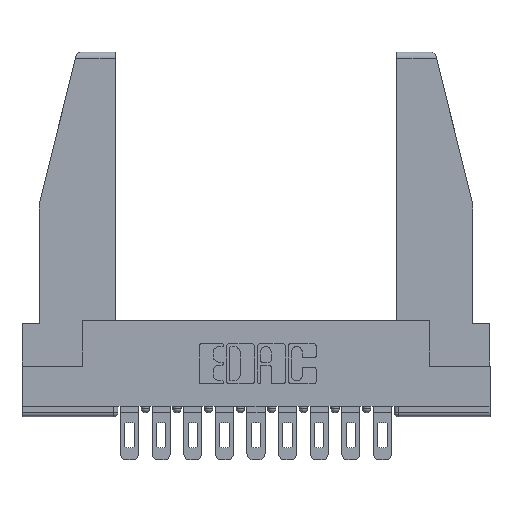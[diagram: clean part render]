
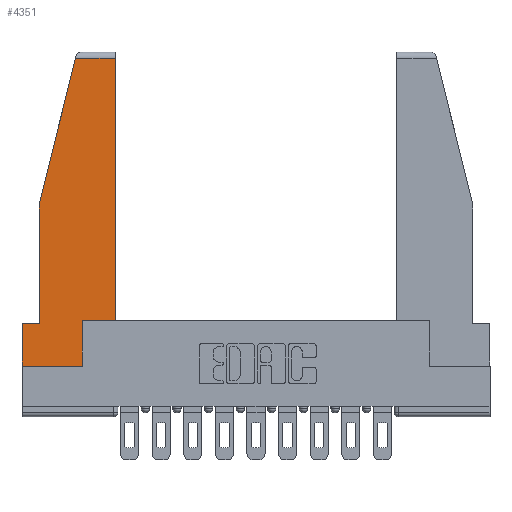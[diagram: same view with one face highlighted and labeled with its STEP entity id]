
A CAD part, top view. The second image highlights one B-rep face of the part: STEP entity #4351.
In plain terms, the highlighted planar face has unit normal (0, 0, 1).
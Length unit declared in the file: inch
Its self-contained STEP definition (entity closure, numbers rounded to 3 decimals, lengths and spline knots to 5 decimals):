
#62 = LINE ( 'NONE', #11621, #13755 ) ;
#148 = CARTESIAN_POINT ( 'NONE',  ( 0.2636, 1.52, 0. ) ) ;
#580 = CARTESIAN_POINT ( 'NONE',  ( 0., 1.52, 0. ) ) ;
#766 = LINE ( 'NONE', #9977, #7907 ) ;
#957 = LINE ( 'NONE', #4331, #13274 ) ;
#1027 = ORIENTED_EDGE ( 'NONE', *, *, #6216, .T. ) ;
#1059 = VERTEX_POINT ( 'NONE', #148 ) ;
#1178 = DIRECTION ( 'NONE',  ( 0., 1., 0. ) ) ;
#1854 = VERTEX_POINT ( 'NONE', #5735 ) ;
#1939 = CARTESIAN_POINT ( 'NONE',  ( 0., 0.21, 0. ) ) ;
#2094 = LINE ( 'NONE', #1939, #12218 ) ;
#2110 = EDGE_LOOP ( 'NONE', ( #8603, #5921, #12155, #1027, #12342, #12570, #11087, #5891, #13607 ) ) ;
#2282 = DIRECTION ( 'NONE',  ( 0., 1., 0. ) ) ;
#3157 = DIRECTION ( 'NONE',  ( -1., 0., 0. ) ) ;
#3195 = DIRECTION ( 'NONE',  ( 0., -1., 0. ) ) ;
#3197 = VECTOR ( 'NONE', #13126, 39.37008 ) ;
#3255 = PLANE ( 'NONE',  #10807 ) ;
#3324 = DIRECTION ( 'NONE',  ( -0.239, -0.971, 0. ) ) ;
#3366 = VERTEX_POINT ( 'NONE', #14363 ) ;
#3514 = CARTESIAN_POINT ( 'NONE',  ( 0.461, 0.223, 0. ) ) ;
#3780 = VERTEX_POINT ( 'NONE', #7477 ) ;
#3920 = VERTEX_POINT ( 'NONE', #4432 ) ;
#3982 = EDGE_CURVE ( 'NONE', #3780, #3366, #766, .T. ) ;
#4331 = CARTESIAN_POINT ( 'NONE',  ( 0.271, 1.55, 0. ) ) ;
#4351 = ADVANCED_FACE ( 'NONE', ( #12247 ), #3255, .T. ) ;
#4432 = CARTESIAN_POINT ( 'NONE',  ( 0.086, 0.8, 0. ) ) ;
#4512 = EDGE_CURVE ( 'NONE', #1854, #13811, #62, .T. ) ;
#4668 = VERTEX_POINT ( 'NONE', #13221 ) ;
#5735 = CARTESIAN_POINT ( 'NONE',  ( 0.297, 0.223, 0. ) ) ;
#5763 = VERTEX_POINT ( 'NONE', #11173 ) ;
#5773 = CARTESIAN_POINT ( 'NONE',  ( 0.461, 0.223, 0. ) ) ;
#5867 = VECTOR ( 'NONE', #13600, 39.37008 ) ;
#5891 = ORIENTED_EDGE ( 'NONE', *, *, #8280, .T. ) ;
#5921 = ORIENTED_EDGE ( 'NONE', *, *, #11559, .T. ) ;
#5927 = DIRECTION ( 'NONE',  ( 1., 0., 0. ) ) ;
#5994 = LINE ( 'NONE', #12912, #12396 ) ;
#6216 = EDGE_CURVE ( 'NONE', #3920, #4668, #9172, .T. ) ;
#6544 = DIRECTION ( 'NONE',  ( 1., 0., 0. ) ) ;
#6897 = EDGE_CURVE ( 'NONE', #1059, #3920, #957, .T. ) ;
#7081 = VECTOR ( 'NONE', #2282, 39.37008 ) ;
#7477 = CARTESIAN_POINT ( 'NONE',  ( 0., 0.21, 0. ) ) ;
#7907 = VECTOR ( 'NONE', #3195, 39.37008 ) ;
#8280 = EDGE_CURVE ( 'NONE', #14817, #1854, #5994, .T. ) ;
#8603 = ORIENTED_EDGE ( 'NONE', *, *, #9186, .T. ) ;
#9172 = LINE ( 'NONE', #13759, #10819 ) ;
#9186 = EDGE_CURVE ( 'NONE', #13811, #5763, #10354, .T. ) ;
#9977 = CARTESIAN_POINT ( 'NONE',  ( 0., 0.21, 0. ) ) ;
#10178 = DIRECTION ( 'NONE',  ( 0., 0., 1. ) ) ;
#10354 = LINE ( 'NONE', #3514, #7081 ) ;
#10378 = DIRECTION ( 'NONE',  ( 0., -1., 0. ) ) ;
#10430 = CARTESIAN_POINT ( 'NONE',  ( 0., 0., 0. ) ) ;
#10807 = AXIS2_PLACEMENT_3D ( 'NONE', #11252, #10178, #6544 ) ;
#10819 = VECTOR ( 'NONE', #10378, 39.37008 ) ;
#11087 = ORIENTED_EDGE ( 'NONE', *, *, #14277, .T. ) ;
#11173 = CARTESIAN_POINT ( 'NONE',  ( 0.461, 1.52, 0. ) ) ;
#11252 = CARTESIAN_POINT ( 'NONE',  ( 0., 0., 0. ) ) ;
#11337 = EDGE_CURVE ( 'NONE', #4668, #3780, #2094, .T. ) ;
#11559 = EDGE_CURVE ( 'NONE', #5763, #1059, #12207, .T. ) ;
#11621 = CARTESIAN_POINT ( 'NONE',  ( 0.297, 0.223, 0. ) ) ;
#12155 = ORIENTED_EDGE ( 'NONE', *, *, #6897, .T. ) ;
#12207 = LINE ( 'NONE', #580, #3197 ) ;
#12218 = VECTOR ( 'NONE', #3157, 39.37008 ) ;
#12247 = FACE_OUTER_BOUND ( 'NONE', #2110, .T. ) ;
#12342 = ORIENTED_EDGE ( 'NONE', *, *, #11337, .T. ) ;
#12396 = VECTOR ( 'NONE', #1178, 39.37008 ) ;
#12570 = ORIENTED_EDGE ( 'NONE', *, *, #3982, .T. ) ;
#12912 = CARTESIAN_POINT ( 'NONE',  ( 0.297, 0., 0. ) ) ;
#13126 = DIRECTION ( 'NONE',  ( -1., 0., 0. ) ) ;
#13221 = CARTESIAN_POINT ( 'NONE',  ( 0.086, 0.21, 0. ) ) ;
#13274 = VECTOR ( 'NONE', #3324, 39.37008 ) ;
#13600 = DIRECTION ( 'NONE',  ( 1., 0., 0. ) ) ;
#13607 = ORIENTED_EDGE ( 'NONE', *, *, #4512, .T. ) ;
#13755 = VECTOR ( 'NONE', #5927, 39.37008 ) ;
#13759 = CARTESIAN_POINT ( 'NONE',  ( 0.086, 0.8, 0. ) ) ;
#13811 = VERTEX_POINT ( 'NONE', #5773 ) ;
#14277 = EDGE_CURVE ( 'NONE', #3366, #14817, #14877, .T. ) ;
#14363 = CARTESIAN_POINT ( 'NONE',  ( 0., 0., 0. ) ) ;
#14747 = CARTESIAN_POINT ( 'NONE',  ( 0.297, 0., 0. ) ) ;
#14817 = VERTEX_POINT ( 'NONE', #14747 ) ;
#14877 = LINE ( 'NONE', #10430, #5867 ) ;
